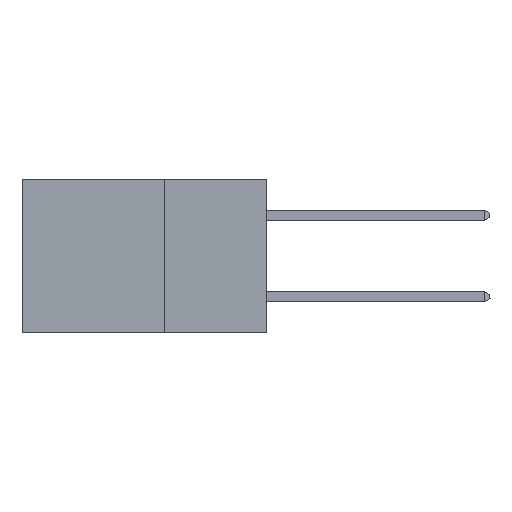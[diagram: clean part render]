
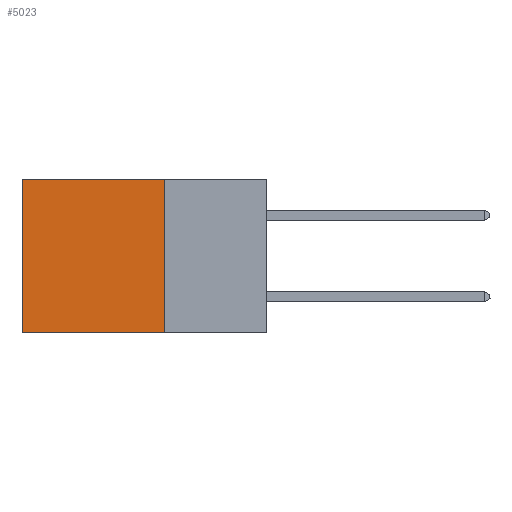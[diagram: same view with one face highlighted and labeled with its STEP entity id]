
A CAD part, left-side view. The second image highlights one B-rep face of the part: STEP entity #5023.
In plain terms, the highlighted planar face has unit normal (-1, 0, 0).
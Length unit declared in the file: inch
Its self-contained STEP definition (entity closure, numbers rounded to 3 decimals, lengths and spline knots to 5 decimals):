
#206 = CARTESIAN_POINT ( 'NONE',  ( 0.2875, 0.25, -0.375 ) ) ;
#272 = ORIENTED_EDGE ( 'NONE', *, *, #15647, .T. ) ;
#1085 = EDGE_CURVE ( 'NONE', #3800, #7133, #5149, .T. ) ;
#1333 = AXIS2_PLACEMENT_3D ( 'NONE', #5413, #1741, #9625 ) ;
#1659 = VECTOR ( 'NONE', #2847, 39.37008 ) ;
#1741 = DIRECTION ( 'NONE',  ( 1., 0., 0. ) ) ;
#2759 = EDGE_CURVE ( 'NONE', #11012, #3800, #8571, .T. ) ;
#2847 = DIRECTION ( 'NONE',  ( 0., 1., 0. ) ) ;
#3464 = ORIENTED_EDGE ( 'NONE', *, *, #7407, .T. ) ;
#3784 = DIRECTION ( 'NONE',  ( 0., 1., 0. ) ) ;
#3800 = VERTEX_POINT ( 'NONE', #7752 ) ;
#4221 = PLANE ( 'NONE',  #1333 ) ;
#4558 = CARTESIAN_POINT ( 'NONE',  ( 0.2875, 0.6, 0. ) ) ;
#5023 = ADVANCED_FACE ( 'NONE', ( #12377 ), #4221, .F. ) ;
#5149 = LINE ( 'NONE', #206, #1659 ) ;
#5413 = CARTESIAN_POINT ( 'NONE',  ( 0.2875, 0.25, -0.375 ) ) ;
#6006 = VERTEX_POINT ( 'NONE', #4558 ) ;
#7133 = VERTEX_POINT ( 'NONE', #11679 ) ;
#7407 = EDGE_CURVE ( 'NONE', #6006, #7133, #8090, .T. ) ;
#7752 = CARTESIAN_POINT ( 'NONE',  ( 0.2875, 0.25, -0.375 ) ) ;
#8090 = LINE ( 'NONE', #9688, #11774 ) ;
#8349 = DIRECTION ( 'NONE',  ( 0., 0., -1. ) ) ;
#8571 = LINE ( 'NONE', #12728, #13458 ) ;
#8757 = EDGE_LOOP ( 'NONE', ( #3464, #13767, #14882, #272 ) ) ;
#9625 = DIRECTION ( 'NONE',  ( 0., 0., -1. ) ) ;
#9688 = CARTESIAN_POINT ( 'NONE',  ( 0.2875, 0.6, -0.375 ) ) ;
#10121 = CARTESIAN_POINT ( 'NONE',  ( 0.2875, 0.25, 0. ) ) ;
#10490 = CARTESIAN_POINT ( 'NONE',  ( 0.2875, 0.25, 0. ) ) ;
#11012 = VERTEX_POINT ( 'NONE', #10490 ) ;
#11679 = CARTESIAN_POINT ( 'NONE',  ( 0.2875, 0.6, -0.375 ) ) ;
#11774 = VECTOR ( 'NONE', #8349, 39.37008 ) ;
#12377 = FACE_OUTER_BOUND ( 'NONE', #8757, .T. ) ;
#12728 = CARTESIAN_POINT ( 'NONE',  ( 0.2875, 0.25, -0.375 ) ) ;
#13458 = VECTOR ( 'NONE', #13977, 39.37008 ) ;
#13767 = ORIENTED_EDGE ( 'NONE', *, *, #1085, .F. ) ;
#13977 = DIRECTION ( 'NONE',  ( 0., 0., -1. ) ) ;
#14114 = LINE ( 'NONE', #10121, #16358 ) ;
#14882 = ORIENTED_EDGE ( 'NONE', *, *, #2759, .F. ) ;
#15647 = EDGE_CURVE ( 'NONE', #11012, #6006, #14114, .T. ) ;
#16358 = VECTOR ( 'NONE', #3784, 39.37008 ) ;
